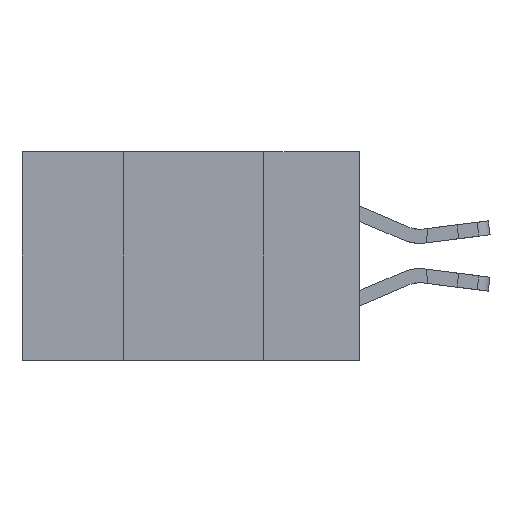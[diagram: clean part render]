
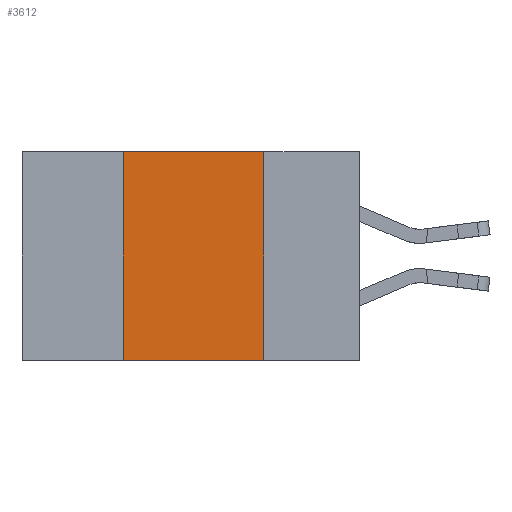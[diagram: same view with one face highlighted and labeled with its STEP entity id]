
A CAD part, left-side view. The second image highlights one B-rep face of the part: STEP entity #3612.
In plain terms, the highlighted planar face has unit normal (-1, 0, 0).
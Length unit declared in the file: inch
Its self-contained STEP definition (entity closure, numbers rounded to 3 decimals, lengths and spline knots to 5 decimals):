
#650 = LINE ( 'NONE', #17914, #1682 ) ;
#833 = CARTESIAN_POINT ( 'NONE',  ( 0., 0.17, -0.37 ) ) ;
#924 = VERTEX_POINT ( 'NONE', #11271 ) ;
#1682 = VECTOR ( 'NONE', #11608, 39.37008 ) ;
#3612 = ADVANCED_FACE ( 'NONE', ( #3806 ), #17012, .F. ) ;
#3806 = FACE_OUTER_BOUND ( 'NONE', #22389, .T. ) ;
#5369 = AXIS2_PLACEMENT_3D ( 'NONE', #14754, #23473, #18923 ) ;
#6791 = DIRECTION ( 'NONE',  ( 0., -1., 0. ) ) ;
#8229 = CARTESIAN_POINT ( 'NONE',  ( 0., 0.42, 0. ) ) ;
#11271 = CARTESIAN_POINT ( 'NONE',  ( 0., 0.17, 0. ) ) ;
#11481 = ORIENTED_EDGE ( 'NONE', *, *, #20242, .F. ) ;
#11608 = DIRECTION ( 'NONE',  ( 0., 0., -1. ) ) ;
#11651 = VECTOR ( 'NONE', #6791, 39.37008 ) ;
#12021 = VERTEX_POINT ( 'NONE', #8229 ) ;
#12046 = ORIENTED_EDGE ( 'NONE', *, *, #25145, .T. ) ;
#12421 = ORIENTED_EDGE ( 'NONE', *, *, #17937, .F. ) ;
#13098 = VERTEX_POINT ( 'NONE', #833 ) ;
#14154 = VECTOR ( 'NONE', #15519, 39.37008 ) ;
#14754 = CARTESIAN_POINT ( 'NONE',  ( 0., 0.6, 0. ) ) ;
#15519 = DIRECTION ( 'NONE',  ( 0., -1., 0. ) ) ;
#15602 = CARTESIAN_POINT ( 'NONE',  ( 0., 0.6, 0. ) ) ;
#15627 = ORIENTED_EDGE ( 'NONE', *, *, #15628, .F. ) ;
#15628 = EDGE_CURVE ( 'NONE', #23679, #12021, #24243, .T. ) ;
#15983 = VECTOR ( 'NONE', #21850, 39.37008 ) ;
#16567 = LINE ( 'NONE', #15602, #14154 ) ;
#17012 = PLANE ( 'NONE',  #5369 ) ;
#17345 = LINE ( 'NONE', #17521, #11651 ) ;
#17521 = CARTESIAN_POINT ( 'NONE',  ( 0., 0.6, -0.37 ) ) ;
#17914 = CARTESIAN_POINT ( 'NONE',  ( 0., 0.17, 0. ) ) ;
#17937 = EDGE_CURVE ( 'NONE', #12021, #924, #16567, .T. ) ;
#18923 = DIRECTION ( 'NONE',  ( 0., 0., -1. ) ) ;
#19691 = CARTESIAN_POINT ( 'NONE',  ( 0., 0.42, 0. ) ) ;
#20242 = EDGE_CURVE ( 'NONE', #924, #13098, #650, .T. ) ;
#20838 = CARTESIAN_POINT ( 'NONE',  ( 0., 0.42, -0.37 ) ) ;
#21850 = DIRECTION ( 'NONE',  ( 0., 0., 1. ) ) ;
#22389 = EDGE_LOOP ( 'NONE', ( #11481, #12421, #15627, #12046 ) ) ;
#23473 = DIRECTION ( 'NONE',  ( 1., 0., 0. ) ) ;
#23679 = VERTEX_POINT ( 'NONE', #20838 ) ;
#24243 = LINE ( 'NONE', #19691, #15983 ) ;
#25145 = EDGE_CURVE ( 'NONE', #23679, #13098, #17345, .T. ) ;
